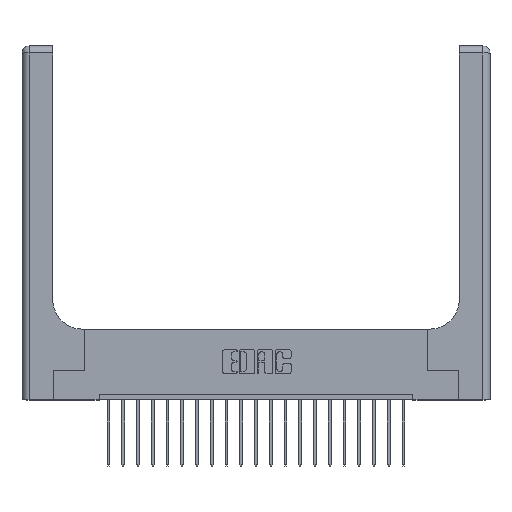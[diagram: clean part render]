
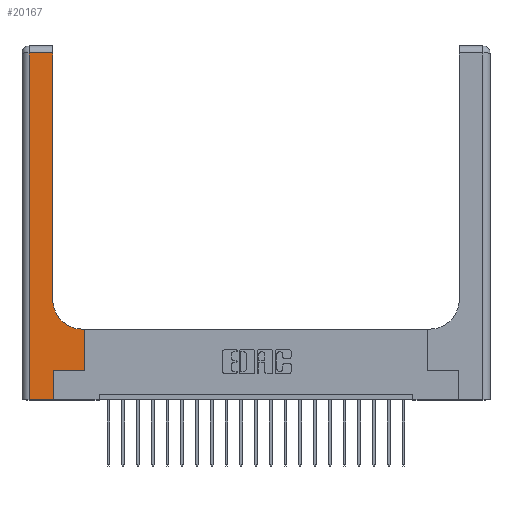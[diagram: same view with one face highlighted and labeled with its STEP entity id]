
A CAD part, top view. The second image highlights one B-rep face of the part: STEP entity #20167.
In plain terms, the highlighted planar face has unit normal (0, 0, 1).
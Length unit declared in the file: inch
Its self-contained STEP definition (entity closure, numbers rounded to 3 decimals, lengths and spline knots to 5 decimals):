
#58 = DIRECTION ( 'NONE',  ( -1., 0., 0. ) ) ;
#133 = VECTOR ( 'NONE', #58, 39.37008 ) ;
#182 = AXIS2_PLACEMENT_3D ( 'NONE', #14857, #5085, #16395 ) ;
#526 = EDGE_CURVE ( 'NONE', #16940, #19968, #12797, .T. ) ;
#817 = EDGE_CURVE ( 'NONE', #4148, #2601, #16047, .T. ) ;
#984 = ORIENTED_EDGE ( 'NONE', *, *, #8653, .T. ) ;
#1530 = CIRCLE ( 'NONE', #15053, 0.25 ) ;
#2323 = CARTESIAN_POINT ( 'NONE',  ( 0.265, 0., 0.37 ) ) ;
#2601 = VERTEX_POINT ( 'NONE', #5039 ) ;
#3393 = EDGE_CURVE ( 'NONE', #19224, #12096, #8526, .T. ) ;
#3509 = VECTOR ( 'NONE', #16155, 39.37008 ) ;
#3636 = CARTESIAN_POINT ( 'NONE',  ( 0.06, 3., 0.37 ) ) ;
#4148 = VERTEX_POINT ( 'NONE', #6108 ) ;
#4277 = LINE ( 'NONE', #14161, #17595 ) ;
#4490 = CARTESIAN_POINT ( 'NONE',  ( 0.51, 0.85, 0.37 ) ) ;
#5039 = CARTESIAN_POINT ( 'NONE',  ( 0.51, 0.6, 0.37 ) ) ;
#5070 = CARTESIAN_POINT ( 'NONE',  ( 0., 0., 0.37 ) ) ;
#5085 = DIRECTION ( 'NONE',  ( 0., 0., -1. ) ) ;
#5546 = ORIENTED_EDGE ( 'NONE', *, *, #3393, .T. ) ;
#5688 = ORIENTED_EDGE ( 'NONE', *, *, #526, .T. ) ;
#5904 = DIRECTION ( 'NONE',  ( 1., 0., 0. ) ) ;
#6108 = CARTESIAN_POINT ( 'NONE',  ( 0.528, 0.6, 0.37 ) ) ;
#6437 = EDGE_CURVE ( 'NONE', #12414, #11141, #13577, .T. ) ;
#6645 = CARTESIAN_POINT ( 'NONE',  ( 0.265, 0., 0.37 ) ) ;
#6969 = VECTOR ( 'NONE', #14155, 39.37008 ) ;
#7082 = CARTESIAN_POINT ( 'NONE',  ( 0.06, 0., 0.37 ) ) ;
#7169 = CARTESIAN_POINT ( 'NONE',  ( 0.265, 0.25, 0.37 ) ) ;
#7503 = LINE ( 'NONE', #3636, #14812 ) ;
#7738 = CARTESIAN_POINT ( 'NONE',  ( 0.528, 0.25, 0.37 ) ) ;
#8403 = LINE ( 'NONE', #16253, #133 ) ;
#8526 = LINE ( 'NONE', #5070, #18253 ) ;
#8547 = DIRECTION ( 'NONE',  ( 0., 1., 0. ) ) ;
#8653 = EDGE_CURVE ( 'NONE', #10540, #19224, #7503, .T. ) ;
#9660 = CARTESIAN_POINT ( 'NONE',  ( 0.06, 2.94, 0.37 ) ) ;
#9858 = PLANE ( 'NONE',  #182 ) ;
#9977 = EDGE_CURVE ( 'NONE', #11141, #4148, #4277, .T. ) ;
#10540 = VERTEX_POINT ( 'NONE', #9660 ) ;
#10931 = CARTESIAN_POINT ( 'NONE',  ( 0.26, 0.6, 0.37 ) ) ;
#11141 = VERTEX_POINT ( 'NONE', #7738 ) ;
#11837 = DIRECTION ( 'NONE',  ( 1., 0., 0. ) ) ;
#11874 = VECTOR ( 'NONE', #8547, 39.37008 ) ;
#11880 = DIRECTION ( 'NONE',  ( 0., -1., 0. ) ) ;
#12096 = VERTEX_POINT ( 'NONE', #6645 ) ;
#12265 = CARTESIAN_POINT ( 'NONE',  ( 0.26, 2.94, 0.37 ) ) ;
#12302 = LINE ( 'NONE', #2323, #6969 ) ;
#12374 = ORIENTED_EDGE ( 'NONE', *, *, #6437, .T. ) ;
#12414 = VERTEX_POINT ( 'NONE', #15377 ) ;
#12797 = LINE ( 'NONE', #15180, #11874 ) ;
#13577 = LINE ( 'NONE', #7169, #17162 ) ;
#13663 = ORIENTED_EDGE ( 'NONE', *, *, #19037, .T. ) ;
#14155 = DIRECTION ( 'NONE',  ( 0., 1., 0. ) ) ;
#14161 = CARTESIAN_POINT ( 'NONE',  ( 0.528, 0.25, 0.37 ) ) ;
#14812 = VECTOR ( 'NONE', #11880, 39.37008 ) ;
#14857 = CARTESIAN_POINT ( 'NONE',  ( 0., 3., 0.37 ) ) ;
#15053 = AXIS2_PLACEMENT_3D ( 'NONE', #4490, #16121, #5904 ) ;
#15065 = CARTESIAN_POINT ( 'NONE',  ( 0.26, 0.85, 0.37 ) ) ;
#15162 = DIRECTION ( 'NONE',  ( 1., 0., 0. ) ) ;
#15180 = CARTESIAN_POINT ( 'NONE',  ( 0.26, 3., 0.37 ) ) ;
#15377 = CARTESIAN_POINT ( 'NONE',  ( 0.265, 0.25, 0.37 ) ) ;
#15608 = EDGE_CURVE ( 'NONE', #12096, #12414, #12302, .T. ) ;
#15748 = FACE_OUTER_BOUND ( 'NONE', #15830, .T. ) ;
#15830 = EDGE_LOOP ( 'NONE', ( #5688, #20241, #984, #5546, #19373, #12374, #20100, #17901, #13663 ) ) ;
#16047 = LINE ( 'NONE', #10931, #3509 ) ;
#16121 = DIRECTION ( 'NONE',  ( 0., 0., -1. ) ) ;
#16155 = DIRECTION ( 'NONE',  ( -1., 0., 0. ) ) ;
#16253 = CARTESIAN_POINT ( 'NONE',  ( 0., 2.94, 0.37 ) ) ;
#16395 = DIRECTION ( 'NONE',  ( -1., 0., 0. ) ) ;
#16940 = VERTEX_POINT ( 'NONE', #15065 ) ;
#17162 = VECTOR ( 'NONE', #11837, 39.37008 ) ;
#17595 = VECTOR ( 'NONE', #17743, 39.37008 ) ;
#17743 = DIRECTION ( 'NONE',  ( 0., 1., 0. ) ) ;
#17901 = ORIENTED_EDGE ( 'NONE', *, *, #817, .T. ) ;
#18253 = VECTOR ( 'NONE', #15162, 39.37008 ) ;
#18680 = EDGE_CURVE ( 'NONE', #19968, #10540, #8403, .T. ) ;
#19037 = EDGE_CURVE ( 'NONE', #2601, #16940, #1530, .T. ) ;
#19224 = VERTEX_POINT ( 'NONE', #7082 ) ;
#19373 = ORIENTED_EDGE ( 'NONE', *, *, #15608, .T. ) ;
#19968 = VERTEX_POINT ( 'NONE', #12265 ) ;
#20100 = ORIENTED_EDGE ( 'NONE', *, *, #9977, .T. ) ;
#20167 = ADVANCED_FACE ( 'NONE', ( #15748 ), #9858, .F. ) ;
#20241 = ORIENTED_EDGE ( 'NONE', *, *, #18680, .T. ) ;
